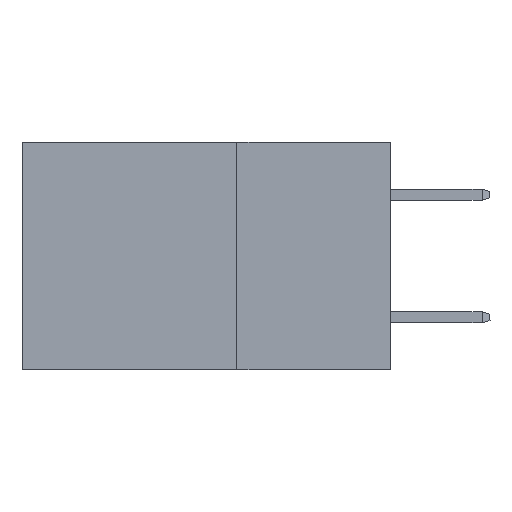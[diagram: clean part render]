
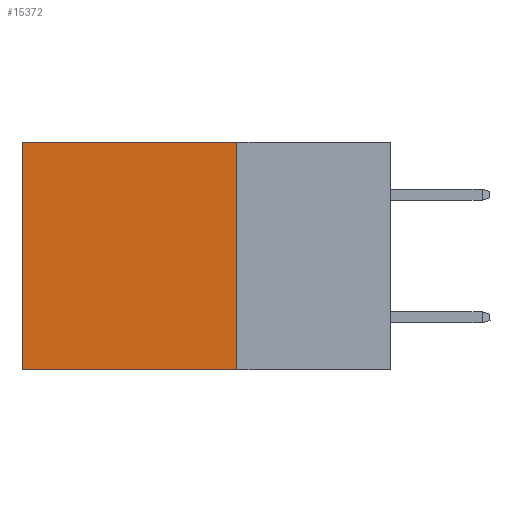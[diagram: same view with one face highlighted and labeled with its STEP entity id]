
A CAD part, left-side view. The second image highlights one B-rep face of the part: STEP entity #15372.
In plain terms, the highlighted planar face has unit normal (-1, 0, 0).
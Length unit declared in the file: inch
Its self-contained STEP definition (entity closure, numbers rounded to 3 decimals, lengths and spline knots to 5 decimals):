
#358 = DIRECTION ( 'NONE',  ( 0., 1., 0. ) ) ;
#704 = CARTESIAN_POINT ( 'NONE',  ( 0.2875, 0.25, 0. ) ) ;
#765 = VECTOR ( 'NONE', #358, 39.37008 ) ;
#1195 = ORIENTED_EDGE ( 'NONE', *, *, #13779, .F. ) ;
#1522 = EDGE_CURVE ( 'NONE', #13898, #11593, #13119, .T. ) ;
#1525 = VECTOR ( 'NONE', #7839, 39.37008 ) ;
#1626 = CARTESIAN_POINT ( 'NONE',  ( 0.2875, 0.25, -0.37 ) ) ;
#4044 = LINE ( 'NONE', #4123, #765 ) ;
#4056 = CARTESIAN_POINT ( 'NONE',  ( 0.2875, 0.6, 0. ) ) ;
#4123 = CARTESIAN_POINT ( 'NONE',  ( 0.2875, 0.25, 0. ) ) ;
#5036 = VECTOR ( 'NONE', #5499, 39.37008 ) ;
#5140 = CARTESIAN_POINT ( 'NONE',  ( 0.2875, 0.25, 0. ) ) ;
#5454 = CARTESIAN_POINT ( 'NONE',  ( 0.2875, 0.6, -0.37 ) ) ;
#5499 = DIRECTION ( 'NONE',  ( 0., 0., -1. ) ) ;
#6068 = CARTESIAN_POINT ( 'NONE',  ( 0.2875, 0.25, -0.37 ) ) ;
#6516 = LINE ( 'NONE', #13050, #5036 ) ;
#7217 = EDGE_CURVE ( 'NONE', #11317, #11593, #15464, .T. ) ;
#7839 = DIRECTION ( 'NONE',  ( 0., 0., -1. ) ) ;
#8850 = PLANE ( 'NONE',  #15510 ) ;
#9227 = EDGE_LOOP ( 'NONE', ( #10735, #9476, #1195, #12559 ) ) ;
#9476 = ORIENTED_EDGE ( 'NONE', *, *, #1522, .F. ) ;
#9669 = CARTESIAN_POINT ( 'NONE',  ( 0.2875, 0.6, 0. ) ) ;
#10735 = ORIENTED_EDGE ( 'NONE', *, *, #7217, .T. ) ;
#10743 = VERTEX_POINT ( 'NONE', #704 ) ;
#11317 = VERTEX_POINT ( 'NONE', #9669 ) ;
#11439 = DIRECTION ( 'NONE',  ( 1., 0., 0. ) ) ;
#11593 = VERTEX_POINT ( 'NONE', #5454 ) ;
#11680 = FACE_OUTER_BOUND ( 'NONE', #9227, .T. ) ;
#11858 = DIRECTION ( 'NONE',  ( 0., 1., 0. ) ) ;
#12559 = ORIENTED_EDGE ( 'NONE', *, *, #14139, .T. ) ;
#13050 = CARTESIAN_POINT ( 'NONE',  ( 0.2875, 0.25, 0. ) ) ;
#13119 = LINE ( 'NONE', #1626, #14143 ) ;
#13779 = EDGE_CURVE ( 'NONE', #10743, #13898, #6516, .T. ) ;
#13898 = VERTEX_POINT ( 'NONE', #6068 ) ;
#14113 = DIRECTION ( 'NONE',  ( 0., 0., -1. ) ) ;
#14139 = EDGE_CURVE ( 'NONE', #10743, #11317, #4044, .T. ) ;
#14143 = VECTOR ( 'NONE', #11858, 39.37008 ) ;
#15372 = ADVANCED_FACE ( 'NONE', ( #11680 ), #8850, .F. ) ;
#15464 = LINE ( 'NONE', #4056, #1525 ) ;
#15510 = AXIS2_PLACEMENT_3D ( 'NONE', #5140, #11439, #14113 ) ;
